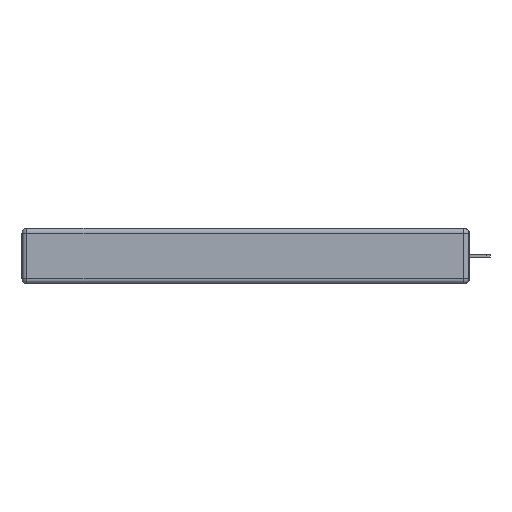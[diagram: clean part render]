
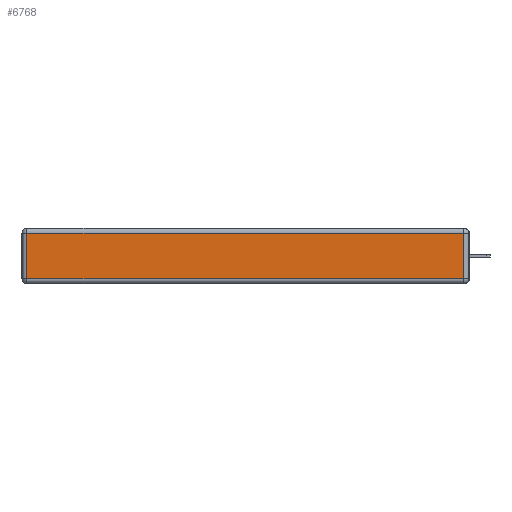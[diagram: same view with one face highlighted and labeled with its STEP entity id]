
A CAD part, left-side view. The second image highlights one B-rep face of the part: STEP entity #6768.
In plain terms, the highlighted planar face has unit normal (-1, 0, 0).
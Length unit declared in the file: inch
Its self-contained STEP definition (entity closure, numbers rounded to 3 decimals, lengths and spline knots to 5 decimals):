
#1 = VERTEX_POINT ( 'NONE', #22354 ) ;
#506 = DIRECTION ( 'NONE',  ( -1., 0., 0. ) ) ;
#632 = DIRECTION ( 'NONE',  ( 0., 0., 1. ) ) ;
#1360 = VECTOR ( 'NONE', #632, 39.37008 ) ;
#2760 = DIRECTION ( 'NONE',  ( 0., 0., -1. ) ) ;
#2795 = FACE_OUTER_BOUND ( 'NONE', #22894, .T. ) ;
#3005 = ORIENTED_EDGE ( 'NONE', *, *, #14601, .T. ) ;
#3644 = EDGE_CURVE ( 'NONE', #20931, #1, #23327, .T. ) ;
#5086 = EDGE_CURVE ( 'NONE', #10270, #20931, #10288, .T. ) ;
#6768 = ADVANCED_FACE ( 'NONE', ( #2795 ), #8576, .T. ) ;
#6935 = VECTOR ( 'NONE', #8226, 39.37008 ) ;
#6957 = VECTOR ( 'NONE', #20582, 39.37008 ) ;
#7571 = LINE ( 'NONE', #18602, #6957 ) ;
#7996 = AXIS2_PLACEMENT_3D ( 'NONE', #12599, #506, #14594 ) ;
#8075 = ORIENTED_EDGE ( 'NONE', *, *, #3644, .T. ) ;
#8226 = DIRECTION ( 'NONE',  ( 0., -1., 0. ) ) ;
#8576 = PLANE ( 'NONE',  #7996 ) ;
#8605 = CARTESIAN_POINT ( 'NONE',  ( 0., 0.03, -0.03 ) ) ;
#8764 = CARTESIAN_POINT ( 'NONE',  ( 0., 2.72, -0.343 ) ) ;
#8895 = ORIENTED_EDGE ( 'NONE', *, *, #5086, .T. ) ;
#10270 = VERTEX_POINT ( 'NONE', #25718 ) ;
#10288 = LINE ( 'NONE', #8764, #14950 ) ;
#12073 = LINE ( 'NONE', #20559, #1360 ) ;
#12245 = CARTESIAN_POINT ( 'NONE',  ( 0., 0., -0.313 ) ) ;
#12599 = CARTESIAN_POINT ( 'NONE',  ( 0., 0., -0.343 ) ) ;
#12994 = CARTESIAN_POINT ( 'NONE',  ( 0., 2.72, -0.313 ) ) ;
#14594 = DIRECTION ( 'NONE',  ( 0., 0., 1. ) ) ;
#14601 = EDGE_CURVE ( 'NONE', #1, #16476, #12073, .T. ) ;
#14950 = VECTOR ( 'NONE', #2760, 39.37008 ) ;
#16476 = VERTEX_POINT ( 'NONE', #8605 ) ;
#18602 = CARTESIAN_POINT ( 'NONE',  ( 0., 2.75, -0.03 ) ) ;
#20559 = CARTESIAN_POINT ( 'NONE',  ( 0., 0.03, -0.343 ) ) ;
#20582 = DIRECTION ( 'NONE',  ( 0., 1., 0. ) ) ;
#20931 = VERTEX_POINT ( 'NONE', #12994 ) ;
#22354 = CARTESIAN_POINT ( 'NONE',  ( 0., 0.03, -0.313 ) ) ;
#22654 = ORIENTED_EDGE ( 'NONE', *, *, #22691, .T. ) ;
#22691 = EDGE_CURVE ( 'NONE', #16476, #10270, #7571, .T. ) ;
#22894 = EDGE_LOOP ( 'NONE', ( #8075, #3005, #22654, #8895 ) ) ;
#23327 = LINE ( 'NONE', #12245, #6935 ) ;
#25718 = CARTESIAN_POINT ( 'NONE',  ( 0., 2.72, -0.03 ) ) ;
